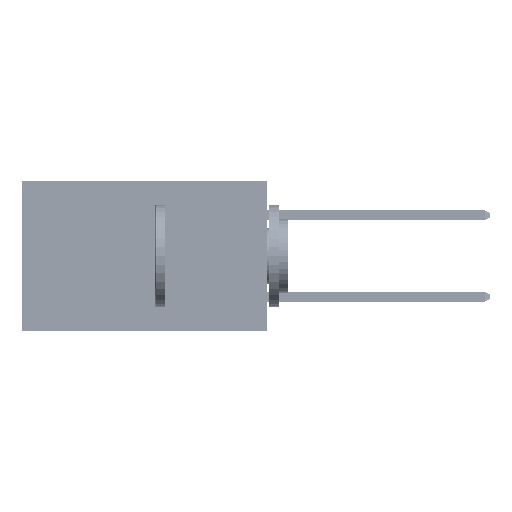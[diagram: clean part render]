
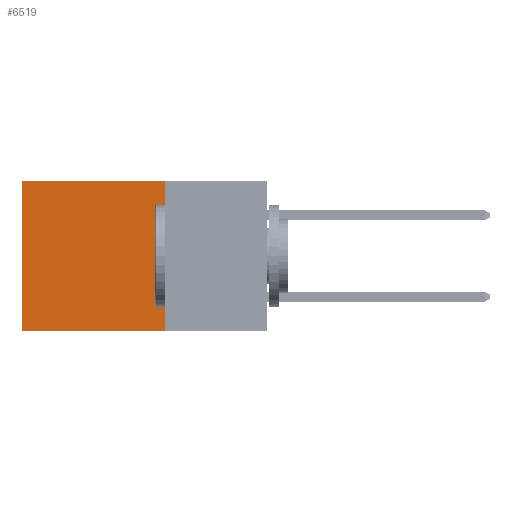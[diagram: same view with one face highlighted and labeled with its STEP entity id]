
A CAD part, left-side view. The second image highlights one B-rep face of the part: STEP entity #6519.
In plain terms, the highlighted planar face has unit normal (-1, 0, 0).
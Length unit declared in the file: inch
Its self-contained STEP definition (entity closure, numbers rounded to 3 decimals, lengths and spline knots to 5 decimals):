
#498 = LINE ( 'NONE', #16401, #29001 ) ;
#3062 = CARTESIAN_POINT ( 'NONE',  ( 0.2875, 0.25, 0. ) ) ;
#3317 = VERTEX_POINT ( 'NONE', #38299 ) ;
#4477 = ORIENTED_EDGE ( 'NONE', *, *, #32351, .T. ) ;
#4568 = ORIENTED_EDGE ( 'NONE', *, *, #7928, .F. ) ;
#6448 = VECTOR ( 'NONE', #7297, 39.37008 ) ;
#6519 = ADVANCED_FACE ( 'NONE', ( #7654 ), #19888, .F. ) ;
#7297 = DIRECTION ( 'NONE',  ( 0., 0., -1. ) ) ;
#7654 = FACE_OUTER_BOUND ( 'NONE', #42739, .T. ) ;
#7865 = DIRECTION ( 'NONE',  ( 1., 0., 0. ) ) ;
#7928 = EDGE_CURVE ( 'NONE', #46840, #29278, #498, .T. ) ;
#8937 = VERTEX_POINT ( 'NONE', #3062 ) ;
#11366 = CARTESIAN_POINT ( 'NONE',  ( 0.2875, 0.6, 0. ) ) ;
#12527 = CARTESIAN_POINT ( 'NONE',  ( 0.2875, 0.6, -0.37 ) ) ;
#15765 = LINE ( 'NONE', #26898, #18283 ) ;
#16401 = CARTESIAN_POINT ( 'NONE',  ( 0.2875, 0.25, -0.37 ) ) ;
#18283 = VECTOR ( 'NONE', #30962, 39.37008 ) ;
#19888 = PLANE ( 'NONE',  #26816 ) ;
#20440 = DIRECTION ( 'NONE',  ( 0., 1., 0. ) ) ;
#26816 = AXIS2_PLACEMENT_3D ( 'NONE', #52348, #7865, #36186 ) ;
#26898 = CARTESIAN_POINT ( 'NONE',  ( 0.2875, 0.25, 0. ) ) ;
#28000 = LINE ( 'NONE', #11366, #6448 ) ;
#28770 = LINE ( 'NONE', #35735, #30016 ) ;
#29001 = VECTOR ( 'NONE', #20440, 39.37008 ) ;
#29124 = EDGE_CURVE ( 'NONE', #8937, #46840, #28770, .T. ) ;
#29278 = VERTEX_POINT ( 'NONE', #12527 ) ;
#30016 = VECTOR ( 'NONE', #51882, 39.37008 ) ;
#30962 = DIRECTION ( 'NONE',  ( 0., 1., 0. ) ) ;
#32351 = EDGE_CURVE ( 'NONE', #8937, #3317, #15765, .T. ) ;
#35735 = CARTESIAN_POINT ( 'NONE',  ( 0.2875, 0.25, 0. ) ) ;
#36186 = DIRECTION ( 'NONE',  ( 0., 0., -1. ) ) ;
#38299 = CARTESIAN_POINT ( 'NONE',  ( 0.2875, 0.6, 0. ) ) ;
#42739 = EDGE_LOOP ( 'NONE', ( #45989, #4568, #48795, #4477 ) ) ;
#45989 = ORIENTED_EDGE ( 'NONE', *, *, #47491, .T. ) ;
#46840 = VERTEX_POINT ( 'NONE', #48077 ) ;
#47491 = EDGE_CURVE ( 'NONE', #3317, #29278, #28000, .T. ) ;
#48077 = CARTESIAN_POINT ( 'NONE',  ( 0.2875, 0.25, -0.37 ) ) ;
#48795 = ORIENTED_EDGE ( 'NONE', *, *, #29124, .F. ) ;
#51882 = DIRECTION ( 'NONE',  ( 0., 0., -1. ) ) ;
#52348 = CARTESIAN_POINT ( 'NONE',  ( 0.2875, 0.25, 0. ) ) ;
